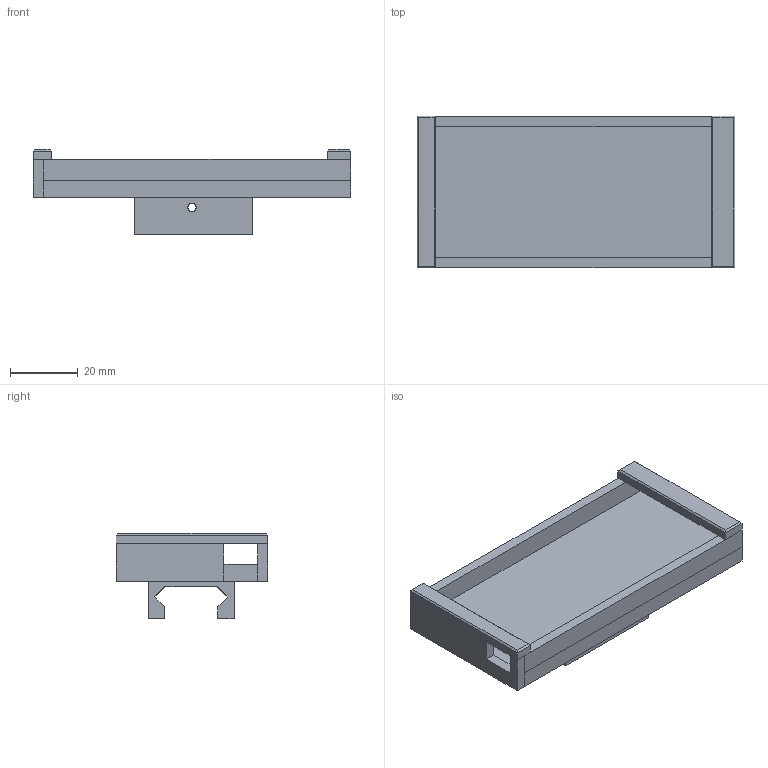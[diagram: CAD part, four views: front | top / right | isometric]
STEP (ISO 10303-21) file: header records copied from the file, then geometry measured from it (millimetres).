
FILE_DESCRIPTION(('Open CASCADE Model'),'2;1');
FILE_NAME('Open CASCADE Shape Model','2013-08-15T18:15:01',('Author'),( 'Open CASCADE'),'Open CASCADE STEP processor 6.5','Open CASCADE 6.5' ,'Unknown');
FILE_SCHEMA(('AUTOMOTIVE_DESIGN_CC2 { 1 2 10303 214 -1 1 5 4 }'));
Length unit declared in the file: millimetre
Products named in the file (1): Cut
Bounding box: 94 x 44.9 x 25.24 mm (x, y, z)
Volume: 30738.6 mm3; surface area: 15796.9 mm2
Topology: 1 solids, 1 shells, 65 faces, 165 edges, 99 vertices
Faces by surface type: plane 63, cylinder 2
Full cylindrical faces by diameter (mm): 2.5 x2
Entity records: 4113 total; most frequent: CARTESIAN_POINT 722, DIRECTION 629, LINE 475, VECTOR 475, ORIENTED_EDGE 330, PCURVE 330, DEFINITIONAL_REPRESENTATION 330, EDGE_CURVE 165
